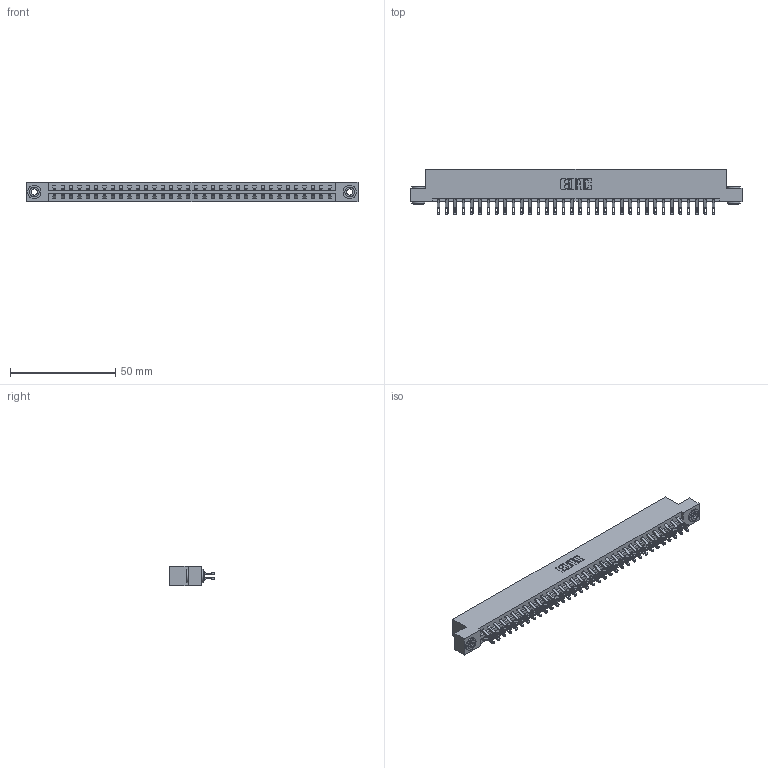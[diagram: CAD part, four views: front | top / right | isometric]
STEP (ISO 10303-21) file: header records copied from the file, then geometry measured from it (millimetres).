
FILE_DESCRIPTION (( 'STEP AP203' ), '1' );
FILE_NAME ('387-068-555-203.STEP', '2019-10-19T21:33:34', ( '' ), ( '' ), 'SwSTEP 2.0', 'SolidWorks 2016', '' );
FILE_SCHEMA (( 'CONFIG_CONTROL_DESIGN' ));
Length unit declared in the file: inch
Products named in the file (4): 345-292-001_555 Tail; 345-250-002_345-250-002-102; 387-068-555-203; 337 Part_Flush Mounting Lugs - 0.156 Dia-TH
Assembly tree (71 placements, depth 2):
  387-068-555-203
    337 Part_Flush Mounting Lugs - 0.156 Dia-TH
    345-292-001_555 Tail  x68
    345-250-002_345-250-002-102  x2
Bounding box: 157.73 x 21.47 x 9.4 mm (x, y, z)
Volume: 16733.4 mm3; surface area: 19807.1 mm2
Topology: 71 solids, 71 shells, 4232 faces, 13239 edges, 8822 vertices
Faces by surface type: plane 2528, cylinder 1696, cone 8
Entity records: 28372 total; most frequent: CARTESIAN_POINT 4795, ORIENTED_EDGE 4694, DIRECTION 4097, EDGE_CURVE 2347, VECTOR 2175, LINE 2175, VERTEX_POINT 1562, AXIS2_PLACEMENT_3D 961
